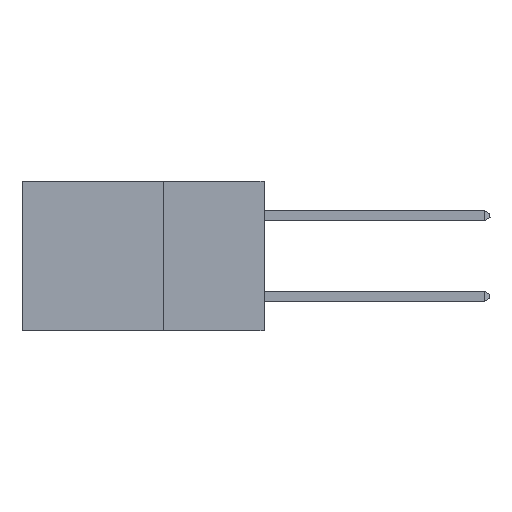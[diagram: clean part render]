
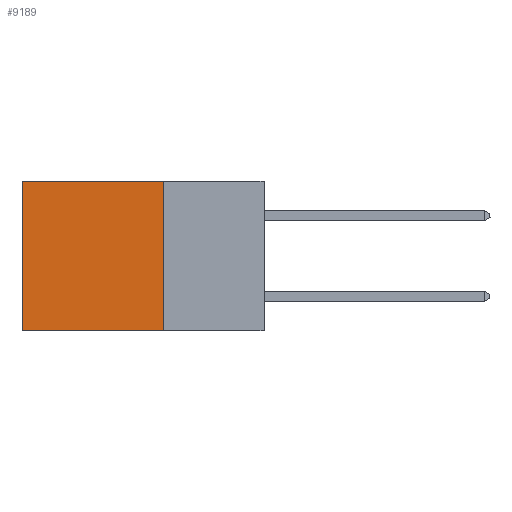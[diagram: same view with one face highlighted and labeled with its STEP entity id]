
A CAD part, left-side view. The second image highlights one B-rep face of the part: STEP entity #9189.
In plain terms, the highlighted planar face has unit normal (-1, 0, 0).
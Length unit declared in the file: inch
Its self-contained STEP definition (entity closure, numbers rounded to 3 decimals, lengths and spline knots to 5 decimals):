
#1756 = VECTOR ( 'NONE', #19848, 39.37008 ) ;
#3214 = ORIENTED_EDGE ( 'NONE', *, *, #15162, .F. ) ;
#3378 = CARTESIAN_POINT ( 'NONE',  ( 0.298, 0.6, 0. ) ) ;
#3603 = EDGE_CURVE ( 'NONE', #19090, #4938, #14220, .T. ) ;
#4044 = PLANE ( 'NONE',  #8604 ) ;
#4938 = VERTEX_POINT ( 'NONE', #3378 ) ;
#5016 = LINE ( 'NONE', #17443, #14556 ) ;
#5327 = CARTESIAN_POINT ( 'NONE',  ( 0.298, 0.6, -0.37 ) ) ;
#5971 = EDGE_CURVE ( 'NONE', #19090, #20077, #17122, .T. ) ;
#6075 = CARTESIAN_POINT ( 'NONE',  ( 0.298, 0.25, 0. ) ) ;
#6857 = LINE ( 'NONE', #8165, #21440 ) ;
#7928 = DIRECTION ( 'NONE',  ( 1., 0., 0. ) ) ;
#8165 = CARTESIAN_POINT ( 'NONE',  ( 0.298, 0.6, 0. ) ) ;
#8604 = AXIS2_PLACEMENT_3D ( 'NONE', #19368, #7928, #21276 ) ;
#9017 = FACE_OUTER_BOUND ( 'NONE', #19698, .T. ) ;
#9189 = ADVANCED_FACE ( 'NONE', ( #9017 ), #4044, .F. ) ;
#10061 = DIRECTION ( 'NONE',  ( 0., 0., -1. ) ) ;
#10762 = EDGE_CURVE ( 'NONE', #4938, #14907, #6857, .T. ) ;
#12604 = CARTESIAN_POINT ( 'NONE',  ( 0.298, 0.25, -0.37 ) ) ;
#14204 = DIRECTION ( 'NONE',  ( 0., 1., 0. ) ) ;
#14220 = LINE ( 'NONE', #16439, #19323 ) ;
#14556 = VECTOR ( 'NONE', #23158, 39.37008 ) ;
#14907 = VERTEX_POINT ( 'NONE', #5327 ) ;
#15162 = EDGE_CURVE ( 'NONE', #20077, #14907, #5016, .T. ) ;
#16439 = CARTESIAN_POINT ( 'NONE',  ( 0.298, 0.25, 0. ) ) ;
#16535 = ORIENTED_EDGE ( 'NONE', *, *, #10762, .T. ) ;
#17122 = LINE ( 'NONE', #18730, #1756 ) ;
#17443 = CARTESIAN_POINT ( 'NONE',  ( 0.298, 0.25, -0.37 ) ) ;
#18730 = CARTESIAN_POINT ( 'NONE',  ( 0.298, 0.25, 0. ) ) ;
#18997 = ORIENTED_EDGE ( 'NONE', *, *, #3603, .T. ) ;
#19090 = VERTEX_POINT ( 'NONE', #6075 ) ;
#19323 = VECTOR ( 'NONE', #14204, 39.37008 ) ;
#19368 = CARTESIAN_POINT ( 'NONE',  ( 0.298, 0.25, 0. ) ) ;
#19698 = EDGE_LOOP ( 'NONE', ( #16535, #3214, #23656, #18997 ) ) ;
#19848 = DIRECTION ( 'NONE',  ( 0., 0., -1. ) ) ;
#20077 = VERTEX_POINT ( 'NONE', #12604 ) ;
#21276 = DIRECTION ( 'NONE',  ( 0., 0., -1. ) ) ;
#21440 = VECTOR ( 'NONE', #10061, 39.37008 ) ;
#23158 = DIRECTION ( 'NONE',  ( 0., 1., 0. ) ) ;
#23656 = ORIENTED_EDGE ( 'NONE', *, *, #5971, .F. ) ;
